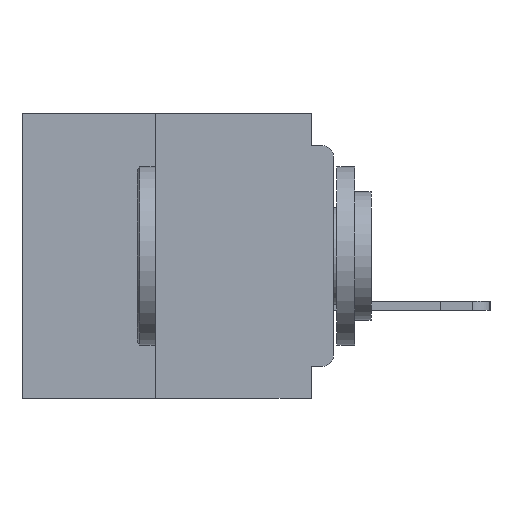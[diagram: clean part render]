
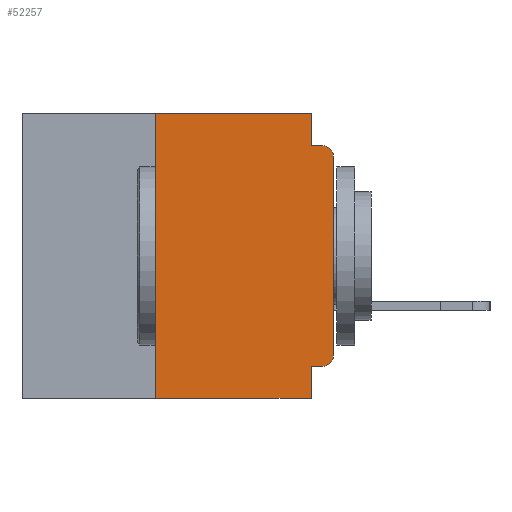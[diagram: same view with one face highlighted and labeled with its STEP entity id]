
A CAD part, left-side view. The second image highlights one B-rep face of the part: STEP entity #52257.
In plain terms, the highlighted planar face has unit normal (-1, 0, 0).
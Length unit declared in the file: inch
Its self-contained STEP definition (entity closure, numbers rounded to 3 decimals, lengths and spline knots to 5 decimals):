
#1240 = VERTEX_POINT ( 'NONE', #42857 ) ;
#2301 = CARTESIAN_POINT ( 'NONE',  ( 0., 0.031, -0.355 ) ) ;
#5223 = EDGE_CURVE ( 'NONE', #38713, #64060, #14623, .T. ) ;
#6737 = LINE ( 'NONE', #20730, #41514 ) ;
#6772 = CARTESIAN_POINT ( 'NONE',  ( 0., 0., -0.355 ) ) ;
#7980 = CARTESIAN_POINT ( 'NONE',  ( 0., 0.437, 0. ) ) ;
#8325 = DIRECTION ( 'NONE',  ( 0., -1., 0. ) ) ;
#8547 = DIRECTION ( 'NONE',  ( -1., 0., 0. ) ) ;
#8834 = ORIENTED_EDGE ( 'NONE', *, *, #28432, .F. ) ;
#9847 = EDGE_CURVE ( 'NONE', #29932, #38713, #6737, .T. ) ;
#10381 = ORIENTED_EDGE ( 'NONE', *, *, #48284, .F. ) ;
#10899 = EDGE_CURVE ( 'NONE', #18222, #1240, #57684, .T. ) ;
#12482 = LINE ( 'NONE', #6772, #63481 ) ;
#12740 = DIRECTION ( 'NONE',  ( -1., 0., 0. ) ) ;
#12983 = PLANE ( 'NONE',  #47923 ) ;
#13484 = VECTOR ( 'NONE', #30185, 39.37008 ) ;
#13607 = VECTOR ( 'NONE', #19038, 39.37008 ) ;
#14623 = CIRCLE ( 'NONE', #51884, 0.015 ) ;
#17954 = DIRECTION ( 'NONE',  ( 0., 0., -1. ) ) ;
#18222 = VERTEX_POINT ( 'NONE', #2301 ) ;
#18518 = CARTESIAN_POINT ( 'NONE',  ( 0., 0.25, 0. ) ) ;
#19038 = DIRECTION ( 'NONE',  ( 0., 0., 1. ) ) ;
#19259 = CARTESIAN_POINT ( 'NONE',  ( 0., 0.25, -0.4 ) ) ;
#20283 = LINE ( 'NONE', #34865, #44987 ) ;
#20404 = ORIENTED_EDGE ( 'NONE', *, *, #9847, .T. ) ;
#20730 = CARTESIAN_POINT ( 'NONE',  ( 0., 0., 0. ) ) ;
#23557 = VECTOR ( 'NONE', #8325, 39.37008 ) ;
#25193 = EDGE_LOOP ( 'NONE', ( #20404, #29475, #37931, #49073, #10381, #56244, #55271, #40312, #8834, #34405 ) ) ;
#25707 = DIRECTION ( 'NONE',  ( 0., 0., 1. ) ) ;
#26085 = VERTEX_POINT ( 'NONE', #53922 ) ;
#26313 = VERTEX_POINT ( 'NONE', #35977 ) ;
#28011 = CARTESIAN_POINT ( 'NONE',  ( 0., 0.437, 0. ) ) ;
#28140 = VECTOR ( 'NONE', #55245, 39.37008 ) ;
#28410 = FACE_OUTER_BOUND ( 'NONE', #25193, .T. ) ;
#28432 = EDGE_CURVE ( 'NONE', #50624, #18222, #12482, .T. ) ;
#29156 = CARTESIAN_POINT ( 'NONE',  ( 0., 0.015, -0.355 ) ) ;
#29475 = ORIENTED_EDGE ( 'NONE', *, *, #5223, .T. ) ;
#29692 = LINE ( 'NONE', #45100, #28140 ) ;
#29932 = VERTEX_POINT ( 'NONE', #34890 ) ;
#30185 = DIRECTION ( 'NONE',  ( 0., 0., -1. ) ) ;
#30990 = DIRECTION ( 'NONE',  ( 0., 0., -1. ) ) ;
#31433 = DIRECTION ( 'NONE',  ( 0., 1., 0. ) ) ;
#34022 = CARTESIAN_POINT ( 'NONE',  ( 0., 0.031, 0. ) ) ;
#34229 = AXIS2_PLACEMENT_3D ( 'NONE', #42314, #12740, #47260 ) ;
#34405 = ORIENTED_EDGE ( 'NONE', *, *, #60216, .T. ) ;
#34865 = CARTESIAN_POINT ( 'NONE',  ( 0., 0., -0.045 ) ) ;
#34890 = CARTESIAN_POINT ( 'NONE',  ( 0., 0., -0.34 ) ) ;
#35977 = CARTESIAN_POINT ( 'NONE',  ( 0., 0.25, -0.4 ) ) ;
#36672 = LINE ( 'NONE', #28011, #23557 ) ;
#37931 = ORIENTED_EDGE ( 'NONE', *, *, #41130, .F. ) ;
#38139 = CARTESIAN_POINT ( 'NONE',  ( 0., 0.015, -0.06 ) ) ;
#38713 = VERTEX_POINT ( 'NONE', #58107 ) ;
#40026 = CIRCLE ( 'NONE', #34229, 0.015 ) ;
#40312 = ORIENTED_EDGE ( 'NONE', *, *, #10899, .F. ) ;
#41026 = VERTEX_POINT ( 'NONE', #34022 ) ;
#41130 = EDGE_CURVE ( 'NONE', #26085, #64060, #20283, .T. ) ;
#41461 = LINE ( 'NONE', #19259, #13607 ) ;
#41514 = VECTOR ( 'NONE', #25707, 39.37008 ) ;
#42314 = CARTESIAN_POINT ( 'NONE',  ( 0., 0.015, -0.34 ) ) ;
#42857 = CARTESIAN_POINT ( 'NONE',  ( 0., 0.031, -0.4 ) ) ;
#43119 = DIRECTION ( 'NONE',  ( 0., 0., -1. ) ) ;
#44545 = VECTOR ( 'NONE', #30990, 39.37008 ) ;
#44987 = VECTOR ( 'NONE', #59491, 39.37008 ) ;
#45100 = CARTESIAN_POINT ( 'NONE',  ( 0., 0.437, -0.4 ) ) ;
#45509 = CARTESIAN_POINT ( 'NONE',  ( 0., 0.015, -0.045 ) ) ;
#45625 = CARTESIAN_POINT ( 'NONE',  ( 0., 0.031, -0.4 ) ) ;
#47260 = DIRECTION ( 'NONE',  ( 0., 0., -1. ) ) ;
#47572 = EDGE_CURVE ( 'NONE', #41026, #26085, #51363, .T. ) ;
#47923 = AXIS2_PLACEMENT_3D ( 'NONE', #7980, #57226, #17954 ) ;
#47970 = EDGE_CURVE ( 'NONE', #26313, #1240, #29692, .T. ) ;
#48284 = EDGE_CURVE ( 'NONE', #58613, #41026, #36672, .T. ) ;
#49073 = ORIENTED_EDGE ( 'NONE', *, *, #47572, .F. ) ;
#50624 = VERTEX_POINT ( 'NONE', #29156 ) ;
#51363 = LINE ( 'NONE', #59759, #13484 ) ;
#51884 = AXIS2_PLACEMENT_3D ( 'NONE', #38139, #8547, #43119 ) ;
#52257 = ADVANCED_FACE ( 'NONE', ( #28410 ), #12983, .F. ) ;
#53922 = CARTESIAN_POINT ( 'NONE',  ( 0., 0.031, -0.045 ) ) ;
#55245 = DIRECTION ( 'NONE',  ( 0., -1., 0. ) ) ;
#55258 = EDGE_CURVE ( 'NONE', #26313, #58613, #41461, .T. ) ;
#55271 = ORIENTED_EDGE ( 'NONE', *, *, #47970, .T. ) ;
#56244 = ORIENTED_EDGE ( 'NONE', *, *, #55258, .F. ) ;
#57226 = DIRECTION ( 'NONE',  ( 1., 0., 0. ) ) ;
#57684 = LINE ( 'NONE', #45625, #44545 ) ;
#58107 = CARTESIAN_POINT ( 'NONE',  ( 0., 0., -0.06 ) ) ;
#58613 = VERTEX_POINT ( 'NONE', #18518 ) ;
#59491 = DIRECTION ( 'NONE',  ( 0., -1., 0. ) ) ;
#59759 = CARTESIAN_POINT ( 'NONE',  ( 0., 0.031, 0. ) ) ;
#60216 = EDGE_CURVE ( 'NONE', #50624, #29932, #40026, .T. ) ;
#63481 = VECTOR ( 'NONE', #31433, 39.37008 ) ;
#64060 = VERTEX_POINT ( 'NONE', #45509 ) ;
